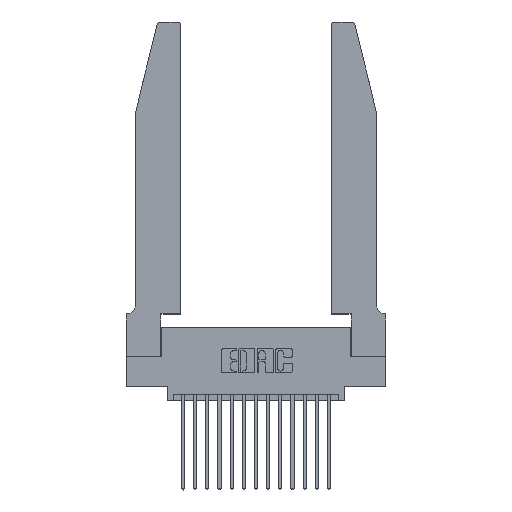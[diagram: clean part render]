
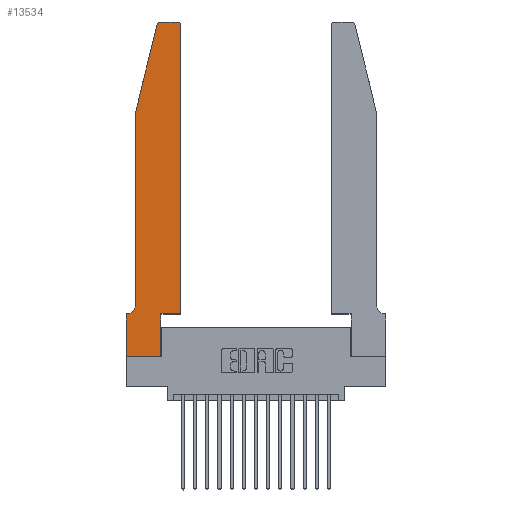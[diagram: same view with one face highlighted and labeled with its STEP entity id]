
A CAD part, top view. The second image highlights one B-rep face of the part: STEP entity #13534.
In plain terms, the highlighted planar face has unit normal (0, 0, 1).
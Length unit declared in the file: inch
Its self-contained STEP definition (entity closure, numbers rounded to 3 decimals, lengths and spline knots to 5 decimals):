
#205 = LINE ( 'NONE', #9274, #7336 ) ;
#300 = EDGE_CURVE ( 'NONE', #9123, #1641, #8915, .T. ) ;
#594 = DIRECTION ( 'NONE',  ( 0., -1., 0. ) ) ;
#969 = ORIENTED_EDGE ( 'NONE', *, *, #11365, .T. ) ;
#977 = EDGE_CURVE ( 'NONE', #4629, #1657, #3422, .T. ) ;
#1031 = CARTESIAN_POINT ( 'NONE',  ( 0.4505, 0.35, 0.37 ) ) ;
#1075 = AXIS2_PLACEMENT_3D ( 'NONE', #2670, #6959, #8444 ) ;
#1141 = VERTEX_POINT ( 'NONE', #1736 ) ;
#1293 = CARTESIAN_POINT ( 'NONE',  ( 0., 0., 0.37 ) ) ;
#1457 = AXIS2_PLACEMENT_3D ( 'NONE', #16532, #3357, #3489 ) ;
#1641 = VERTEX_POINT ( 'NONE', #5947 ) ;
#1657 = VERTEX_POINT ( 'NONE', #7716 ) ;
#1736 = CARTESIAN_POINT ( 'NONE',  ( 0.4505, 2.72, 0.37 ) ) ;
#2334 = VECTOR ( 'NONE', #594, 39.37008 ) ;
#2539 = EDGE_CURVE ( 'NONE', #7437, #10023, #5627, .T. ) ;
#2670 = CARTESIAN_POINT ( 'NONE',  ( 0.0055, 0.42, 0.37 ) ) ;
#2700 = VERTEX_POINT ( 'NONE', #7964 ) ;
#2876 = EDGE_CURVE ( 'NONE', #10023, #17726, #3070, .T. ) ;
#3070 = LINE ( 'NONE', #8469, #9510 ) ;
#3298 = FACE_OUTER_BOUND ( 'NONE', #17920, .T. ) ;
#3357 = DIRECTION ( 'NONE',  ( 0., 0., 1. ) ) ;
#3422 = LINE ( 'NONE', #13109, #16739 ) ;
#3436 = DIRECTION ( 'NONE',  ( -1., 0., 0. ) ) ;
#3489 = DIRECTION ( 'NONE',  ( 1., 0., 0. ) ) ;
#3503 = LINE ( 'NONE', #12226, #18641 ) ;
#3781 = LINE ( 'NONE', #1293, #15483 ) ;
#4557 = CARTESIAN_POINT ( 'NONE',  ( 0., 0.35, 0.37 ) ) ;
#4629 = VERTEX_POINT ( 'NONE', #14718 ) ;
#4945 = CARTESIAN_POINT ( 'NONE',  ( 0.25487, 2.72718, 0.37 ) ) ;
#5396 = ORIENTED_EDGE ( 'NONE', *, *, #977, .T. ) ;
#5627 = CIRCLE ( 'NONE', #1457, 0.03 ) ;
#5666 = CIRCLE ( 'NONE', #8562, 0.03 ) ;
#5763 = ORIENTED_EDGE ( 'NONE', *, *, #17629, .T. ) ;
#5823 = VECTOR ( 'NONE', #12970, 39.37008 ) ;
#5947 = CARTESIAN_POINT ( 'NONE',  ( 0.0055, 0.35, 0.37 ) ) ;
#6246 = CARTESIAN_POINT ( 'NONE',  ( 0.0755, 2., 0.37 ) ) ;
#6959 = DIRECTION ( 'NONE',  ( 0., 0., -1. ) ) ;
#6992 = CARTESIAN_POINT ( 'NONE',  ( 0.284, 2.75, 0.37 ) ) ;
#6994 = DIRECTION ( 'NONE',  ( 1., 0., 0. ) ) ;
#7336 = VECTOR ( 'NONE', #3436, 39.37008 ) ;
#7405 = DIRECTION ( 'NONE',  ( 0., 0., 1. ) ) ;
#7437 = VERTEX_POINT ( 'NONE', #6992 ) ;
#7460 = VERTEX_POINT ( 'NONE', #1031 ) ;
#7483 = ORIENTED_EDGE ( 'NONE', *, *, #2539, .T. ) ;
#7716 = CARTESIAN_POINT ( 'NONE',  ( 0.2865, 0.35, 0.37 ) ) ;
#7964 = CARTESIAN_POINT ( 'NONE',  ( 0.4205, 2.75, 0.37 ) ) ;
#7969 = CARTESIAN_POINT ( 'NONE',  ( 0.0755, 2., 0.37 ) ) ;
#8444 = DIRECTION ( 'NONE',  ( -1., 0., 0. ) ) ;
#8469 = CARTESIAN_POINT ( 'NONE',  ( 0.0755, 2., 0.37 ) ) ;
#8562 = AXIS2_PLACEMENT_3D ( 'NONE', #13253, #7405, #15439 ) ;
#8915 = CIRCLE ( 'NONE', #1075, 0.07 ) ;
#8984 = EDGE_CURVE ( 'NONE', #1641, #13076, #205, .T. ) ;
#9123 = VERTEX_POINT ( 'NONE', #18693 ) ;
#9274 = CARTESIAN_POINT ( 'NONE',  ( 0.0755, 0.35, 0.37 ) ) ;
#9510 = VECTOR ( 'NONE', #11432, 39.37008 ) ;
#10023 = VERTEX_POINT ( 'NONE', #4945 ) ;
#10355 = ORIENTED_EDGE ( 'NONE', *, *, #8984, .T. ) ;
#11365 = EDGE_CURVE ( 'NONE', #1141, #2700, #5666, .T. ) ;
#11391 = CARTESIAN_POINT ( 'NONE',  ( 0., 0., 0.37 ) ) ;
#11395 = EDGE_CURVE ( 'NONE', #7460, #1141, #15313, .T. ) ;
#11422 = EDGE_CURVE ( 'NONE', #2700, #7437, #16002, .T. ) ;
#11432 = DIRECTION ( 'NONE',  ( -0.239, -0.971, 0. ) ) ;
#11924 = VERTEX_POINT ( 'NONE', #11391 ) ;
#12030 = LINE ( 'NONE', #14372, #5823 ) ;
#12226 = CARTESIAN_POINT ( 'NONE',  ( 0.4505, 0.35, 0.37 ) ) ;
#12970 = DIRECTION ( 'NONE',  ( 0., -1., 0. ) ) ;
#13035 = DIRECTION ( 'NONE',  ( 1., 0., 0. ) ) ;
#13076 = VERTEX_POINT ( 'NONE', #4557 ) ;
#13095 = ORIENTED_EDGE ( 'NONE', *, *, #17810, .T. ) ;
#13109 = CARTESIAN_POINT ( 'NONE',  ( 0.2865, 0.35, 0.37 ) ) ;
#13253 = CARTESIAN_POINT ( 'NONE',  ( 0.4205, 2.72, 0.37 ) ) ;
#13329 = EDGE_CURVE ( 'NONE', #13076, #11924, #12030, .T. ) ;
#13364 = EDGE_CURVE ( 'NONE', #11924, #4629, #3781, .T. ) ;
#13430 = ORIENTED_EDGE ( 'NONE', *, *, #11422, .T. ) ;
#13500 = DIRECTION ( 'NONE',  ( 1., 0., 0. ) ) ;
#13534 = ADVANCED_FACE ( 'NONE', ( #3298 ), #15807, .T. ) ;
#14240 = AXIS2_PLACEMENT_3D ( 'NONE', #14248, #15741, #6994 ) ;
#14248 = CARTESIAN_POINT ( 'NONE',  ( 0., 0.35, 0.37 ) ) ;
#14372 = CARTESIAN_POINT ( 'NONE',  ( 0., 0., 0.37 ) ) ;
#14397 = DIRECTION ( 'NONE',  ( -1., 0., 0. ) ) ;
#14718 = CARTESIAN_POINT ( 'NONE',  ( 0.2865, 0., 0.37 ) ) ;
#14835 = VECTOR ( 'NONE', #15712, 39.37008 ) ;
#15035 = ORIENTED_EDGE ( 'NONE', *, *, #2876, .T. ) ;
#15313 = LINE ( 'NONE', #15650, #14835 ) ;
#15439 = DIRECTION ( 'NONE',  ( 1., 0., 0. ) ) ;
#15483 = VECTOR ( 'NONE', #13035, 39.37008 ) ;
#15650 = CARTESIAN_POINT ( 'NONE',  ( 0.4505, 0.35, 0.37 ) ) ;
#15712 = DIRECTION ( 'NONE',  ( 0., 1., 0. ) ) ;
#15741 = DIRECTION ( 'NONE',  ( 0., 0., 1. ) ) ;
#15807 = PLANE ( 'NONE',  #14240 ) ;
#16002 = LINE ( 'NONE', #16096, #18736 ) ;
#16096 = CARTESIAN_POINT ( 'NONE',  ( 0.2605, 2.75, 0.37 ) ) ;
#16476 = ORIENTED_EDGE ( 'NONE', *, *, #11395, .T. ) ;
#16532 = CARTESIAN_POINT ( 'NONE',  ( 0.284, 2.72, 0.37 ) ) ;
#16739 = VECTOR ( 'NONE', #17103, 39.37008 ) ;
#16897 = ORIENTED_EDGE ( 'NONE', *, *, #13329, .T. ) ;
#17103 = DIRECTION ( 'NONE',  ( 0., 1., 0. ) ) ;
#17246 = LINE ( 'NONE', #7969, #2334 ) ;
#17629 = EDGE_CURVE ( 'NONE', #1657, #7460, #3503, .T. ) ;
#17714 = ORIENTED_EDGE ( 'NONE', *, *, #300, .T. ) ;
#17726 = VERTEX_POINT ( 'NONE', #6246 ) ;
#17810 = EDGE_CURVE ( 'NONE', #17726, #9123, #17246, .T. ) ;
#17920 = EDGE_LOOP ( 'NONE', ( #13430, #7483, #15035, #13095, #17714, #10355, #16897, #18668, #5396, #5763, #16476, #969 ) ) ;
#18641 = VECTOR ( 'NONE', #13500, 39.37008 ) ;
#18668 = ORIENTED_EDGE ( 'NONE', *, *, #13364, .T. ) ;
#18693 = CARTESIAN_POINT ( 'NONE',  ( 0.0755, 0.42, 0.37 ) ) ;
#18736 = VECTOR ( 'NONE', #14397, 39.37008 ) ;
